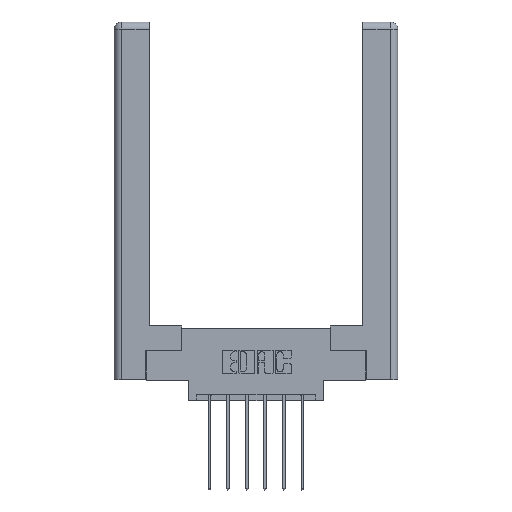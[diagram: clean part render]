
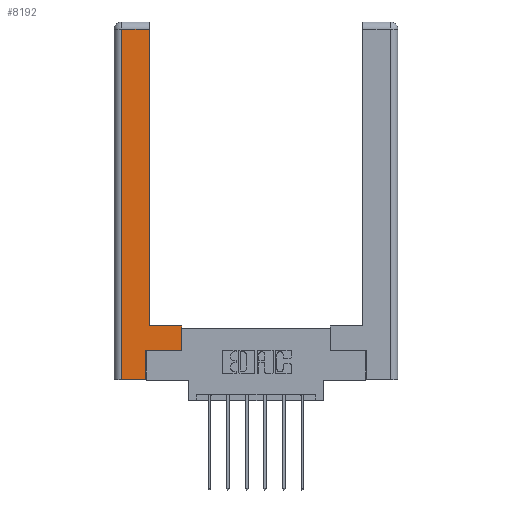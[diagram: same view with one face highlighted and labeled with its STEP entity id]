
A CAD part, top view. The second image highlights one B-rep face of the part: STEP entity #8192.
In plain terms, the highlighted planar face has unit normal (0, 0, 1).
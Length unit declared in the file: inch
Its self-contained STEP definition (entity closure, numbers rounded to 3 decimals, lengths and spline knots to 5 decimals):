
#478 = ORIENTED_EDGE ( 'NONE', *, *, #5515, .T. ) ;
#494 = DIRECTION ( 'NONE',  ( 0., 1., 0. ) ) ;
#860 = VECTOR ( 'NONE', #1951, 39.37008 ) ;
#879 = CARTESIAN_POINT ( 'NONE',  ( 0.295, 3., 0. ) ) ;
#1179 = DIRECTION ( 'NONE',  ( 0., 0., -1. ) ) ;
#1224 = LINE ( 'NONE', #4608, #2711 ) ;
#1233 = VECTOR ( 'NONE', #494, 39.37008 ) ;
#1239 = CARTESIAN_POINT ( 'NONE',  ( 0.0615, 2.94, 0. ) ) ;
#1291 = LINE ( 'NONE', #8736, #10273 ) ;
#1331 = ORIENTED_EDGE ( 'NONE', *, *, #11687, .T. ) ;
#1594 = FACE_OUTER_BOUND ( 'NONE', #2350, .T. ) ;
#1670 = VERTEX_POINT ( 'NONE', #4791 ) ;
#1951 = DIRECTION ( 'NONE',  ( 0., 1., 0. ) ) ;
#2050 = CARTESIAN_POINT ( 'NONE',  ( 0., 0., 0. ) ) ;
#2201 = VECTOR ( 'NONE', #10609, 39.37008 ) ;
#2274 = VECTOR ( 'NONE', #5024, 39.37008 ) ;
#2291 = VERTEX_POINT ( 'NONE', #10373 ) ;
#2310 = CARTESIAN_POINT ( 'NONE',  ( 0.295, 0.45, 0. ) ) ;
#2350 = EDGE_LOOP ( 'NONE', ( #3014, #478, #7744, #7819, #3523, #11005, #10611, #1331 ) ) ;
#2394 = VERTEX_POINT ( 'NONE', #7537 ) ;
#2433 = AXIS2_PLACEMENT_3D ( 'NONE', #2050, #1179, #7786 ) ;
#2511 = CARTESIAN_POINT ( 'NONE',  ( 0.265, 0.245, 0. ) ) ;
#2645 = EDGE_CURVE ( 'NONE', #6634, #2291, #2727, .T. ) ;
#2711 = VECTOR ( 'NONE', #8680, 39.37008 ) ;
#2727 = LINE ( 'NONE', #10703, #2274 ) ;
#3014 = ORIENTED_EDGE ( 'NONE', *, *, #7010, .T. ) ;
#3523 = ORIENTED_EDGE ( 'NONE', *, *, #7939, .T. ) ;
#3751 = CARTESIAN_POINT ( 'NONE',  ( 0.0615, 2.94, 0. ) ) ;
#4387 = LINE ( 'NONE', #879, #860 ) ;
#4608 = CARTESIAN_POINT ( 'NONE',  ( 0.295, 0.45, 0. ) ) ;
#4675 = LINE ( 'NONE', #2511, #8669 ) ;
#4791 = CARTESIAN_POINT ( 'NONE',  ( 0.295, 2.94, 0. ) ) ;
#4864 = VERTEX_POINT ( 'NONE', #7953 ) ;
#5024 = DIRECTION ( 'NONE',  ( 1., 0., 0. ) ) ;
#5096 = LINE ( 'NONE', #8798, #8645 ) ;
#5515 = EDGE_CURVE ( 'NONE', #1670, #6517, #6044, .T. ) ;
#5818 = LINE ( 'NONE', #9088, #1233 ) ;
#6044 = LINE ( 'NONE', #3751, #2201 ) ;
#6491 = EDGE_CURVE ( 'NONE', #6517, #6634, #1291, .T. ) ;
#6517 = VERTEX_POINT ( 'NONE', #1239 ) ;
#6634 = VERTEX_POINT ( 'NONE', #8478 ) ;
#7010 = EDGE_CURVE ( 'NONE', #8804, #1670, #4387, .T. ) ;
#7084 = DIRECTION ( 'NONE',  ( 0., 1., 0. ) ) ;
#7537 = CARTESIAN_POINT ( 'NONE',  ( 0.265, 0.245, 0. ) ) ;
#7744 = ORIENTED_EDGE ( 'NONE', *, *, #6491, .T. ) ;
#7786 = DIRECTION ( 'NONE',  ( -1., 0., 0. ) ) ;
#7819 = ORIENTED_EDGE ( 'NONE', *, *, #2645, .T. ) ;
#7939 = EDGE_CURVE ( 'NONE', #2291, #2394, #4675, .T. ) ;
#7953 = CARTESIAN_POINT ( 'NONE',  ( 0.565, 0.45, 0. ) ) ;
#8192 = ADVANCED_FACE ( 'NONE', ( #1594 ), #10534, .F. ) ;
#8478 = CARTESIAN_POINT ( 'NONE',  ( 0.0615, 0., 0. ) ) ;
#8645 = VECTOR ( 'NONE', #10710, 39.37008 ) ;
#8669 = VECTOR ( 'NONE', #7084, 39.37008 ) ;
#8680 = DIRECTION ( 'NONE',  ( -1., 0., 0. ) ) ;
#8736 = CARTESIAN_POINT ( 'NONE',  ( 0.0615, 0., 0. ) ) ;
#8798 = CARTESIAN_POINT ( 'NONE',  ( 0.565, 0.245, 0. ) ) ;
#8804 = VERTEX_POINT ( 'NONE', #2310 ) ;
#9088 = CARTESIAN_POINT ( 'NONE',  ( 0.565, 0.45, 0. ) ) ;
#9764 = DIRECTION ( 'NONE',  ( 0., -1., 0. ) ) ;
#10016 = EDGE_CURVE ( 'NONE', #2394, #10186, #5096, .T. ) ;
#10186 = VERTEX_POINT ( 'NONE', #11413 ) ;
#10273 = VECTOR ( 'NONE', #9764, 39.37008 ) ;
#10373 = CARTESIAN_POINT ( 'NONE',  ( 0.265, 0., 0. ) ) ;
#10534 = PLANE ( 'NONE',  #2433 ) ;
#10609 = DIRECTION ( 'NONE',  ( -1., 0., 0. ) ) ;
#10611 = ORIENTED_EDGE ( 'NONE', *, *, #11412, .T. ) ;
#10703 = CARTESIAN_POINT ( 'NONE',  ( 0.265, 0., 0. ) ) ;
#10710 = DIRECTION ( 'NONE',  ( 1., 0., 0. ) ) ;
#11005 = ORIENTED_EDGE ( 'NONE', *, *, #10016, .T. ) ;
#11412 = EDGE_CURVE ( 'NONE', #10186, #4864, #5818, .T. ) ;
#11413 = CARTESIAN_POINT ( 'NONE',  ( 0.565, 0.245, 0. ) ) ;
#11687 = EDGE_CURVE ( 'NONE', #4864, #8804, #1224, .T. ) ;
